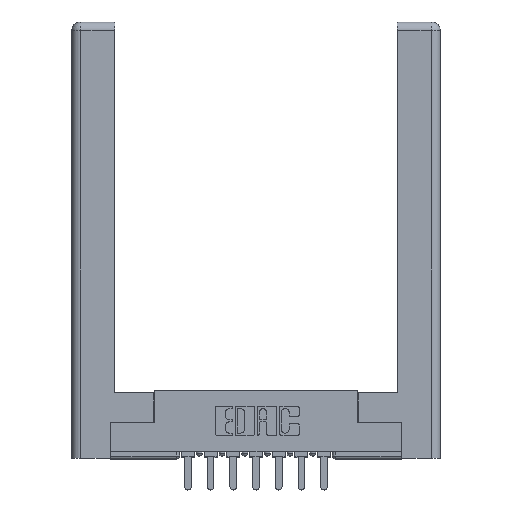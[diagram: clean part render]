
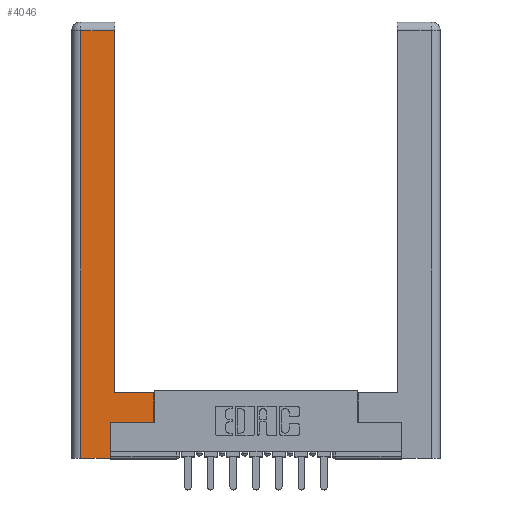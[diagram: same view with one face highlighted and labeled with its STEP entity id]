
A CAD part, top view. The second image highlights one B-rep face of the part: STEP entity #4046.
In plain terms, the highlighted planar face has unit normal (0, 0, 1).
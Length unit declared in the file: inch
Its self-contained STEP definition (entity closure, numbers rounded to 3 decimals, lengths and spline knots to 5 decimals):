
#671 = CARTESIAN_POINT ( 'NONE',  ( 0., 0., 0. ) ) ;
#1032 = VECTOR ( 'NONE', #11446, 39.37008 ) ;
#1261 = VERTEX_POINT ( 'NONE', #8111 ) ;
#1289 = EDGE_CURVE ( 'NONE', #1261, #2173, #3380, .T. ) ;
#1512 = CARTESIAN_POINT ( 'NONE',  ( 0.565, 0.45, 0. ) ) ;
#1563 = FACE_OUTER_BOUND ( 'NONE', #9582, .T. ) ;
#2034 = CARTESIAN_POINT ( 'NONE',  ( 0.565, 0.245, 0. ) ) ;
#2173 = VERTEX_POINT ( 'NONE', #6510 ) ;
#2252 = VERTEX_POINT ( 'NONE', #1512 ) ;
#2338 = ORIENTED_EDGE ( 'NONE', *, *, #1289, .T. ) ;
#2406 = ORIENTED_EDGE ( 'NONE', *, *, #3808, .T. ) ;
#2448 = ORIENTED_EDGE ( 'NONE', *, *, #5752, .T. ) ;
#2510 = LINE ( 'NONE', #8804, #9296 ) ;
#2558 = DIRECTION ( 'NONE',  ( -1., 0., 0. ) ) ;
#2727 = LINE ( 'NONE', #11170, #12758 ) ;
#3006 = LINE ( 'NONE', #4801, #8708 ) ;
#3030 = ORIENTED_EDGE ( 'NONE', *, *, #5508, .T. ) ;
#3164 = VECTOR ( 'NONE', #12103, 39.37008 ) ;
#3380 = LINE ( 'NONE', #12599, #9649 ) ;
#3808 = EDGE_CURVE ( 'NONE', #2252, #13091, #12413, .T. ) ;
#4046 = ADVANCED_FACE ( 'NONE', ( #1563 ), #8781, .F. ) ;
#4602 = CARTESIAN_POINT ( 'NONE',  ( 0.295, 0.45, 0. ) ) ;
#4801 = CARTESIAN_POINT ( 'NONE',  ( 0.0615, 2.94, 0. ) ) ;
#5063 = DIRECTION ( 'NONE',  ( 0., -1., 0. ) ) ;
#5065 = DIRECTION ( 'NONE',  ( 1., 0., 0. ) ) ;
#5245 = EDGE_CURVE ( 'NONE', #2173, #11955, #7089, .T. ) ;
#5508 = EDGE_CURVE ( 'NONE', #11955, #2252, #2510, .T. ) ;
#5752 = EDGE_CURVE ( 'NONE', #6782, #6226, #2727, .T. ) ;
#6035 = CARTESIAN_POINT ( 'NONE',  ( 0.265, 0., 0. ) ) ;
#6226 = VERTEX_POINT ( 'NONE', #11432 ) ;
#6386 = CARTESIAN_POINT ( 'NONE',  ( 0.0615, 2.94, 0. ) ) ;
#6510 = CARTESIAN_POINT ( 'NONE',  ( 0.265, 0.245, 0. ) ) ;
#6622 = CARTESIAN_POINT ( 'NONE',  ( 0.295, 3., 0. ) ) ;
#6713 = ORIENTED_EDGE ( 'NONE', *, *, #10394, .T. ) ;
#6782 = VERTEX_POINT ( 'NONE', #6386 ) ;
#6905 = DIRECTION ( 'NONE',  ( 0., 0., -1. ) ) ;
#7023 = EDGE_CURVE ( 'NONE', #6226, #1261, #11310, .T. ) ;
#7089 = LINE ( 'NONE', #2034, #7773 ) ;
#7704 = AXIS2_PLACEMENT_3D ( 'NONE', #671, #6905, #2558 ) ;
#7773 = VECTOR ( 'NONE', #11322, 39.37008 ) ;
#7911 = CARTESIAN_POINT ( 'NONE',  ( 0.565, 0.245, 0. ) ) ;
#7975 = CARTESIAN_POINT ( 'NONE',  ( 0.295, 2.94, 0. ) ) ;
#7979 = DIRECTION ( 'NONE',  ( 0., 1., 0. ) ) ;
#8111 = CARTESIAN_POINT ( 'NONE',  ( 0.265, 0., 0. ) ) ;
#8347 = ORIENTED_EDGE ( 'NONE', *, *, #5245, .T. ) ;
#8708 = VECTOR ( 'NONE', #13468, 39.37008 ) ;
#8781 = PLANE ( 'NONE',  #7704 ) ;
#8804 = CARTESIAN_POINT ( 'NONE',  ( 0.565, 0.45, 0. ) ) ;
#9127 = EDGE_CURVE ( 'NONE', #13091, #10915, #11062, .T. ) ;
#9296 = VECTOR ( 'NONE', #7979, 39.37008 ) ;
#9582 = EDGE_LOOP ( 'NONE', ( #9651, #6713, #2448, #11566, #2338, #8347, #3030, #2406 ) ) ;
#9649 = VECTOR ( 'NONE', #12734, 39.37008 ) ;
#9651 = ORIENTED_EDGE ( 'NONE', *, *, #9127, .T. ) ;
#10394 = EDGE_CURVE ( 'NONE', #10915, #6782, #3006, .T. ) ;
#10407 = VECTOR ( 'NONE', #5065, 39.37008 ) ;
#10915 = VERTEX_POINT ( 'NONE', #7975 ) ;
#11062 = LINE ( 'NONE', #6622, #3164 ) ;
#11170 = CARTESIAN_POINT ( 'NONE',  ( 0.0615, 0., 0. ) ) ;
#11310 = LINE ( 'NONE', #6035, #10407 ) ;
#11322 = DIRECTION ( 'NONE',  ( 1., 0., 0. ) ) ;
#11432 = CARTESIAN_POINT ( 'NONE',  ( 0.0615, 0., 0. ) ) ;
#11446 = DIRECTION ( 'NONE',  ( -1., 0., 0. ) ) ;
#11566 = ORIENTED_EDGE ( 'NONE', *, *, #7023, .T. ) ;
#11955 = VERTEX_POINT ( 'NONE', #7911 ) ;
#12103 = DIRECTION ( 'NONE',  ( 0., 1., 0. ) ) ;
#12413 = LINE ( 'NONE', #12477, #1032 ) ;
#12477 = CARTESIAN_POINT ( 'NONE',  ( 0.295, 0.45, 0. ) ) ;
#12599 = CARTESIAN_POINT ( 'NONE',  ( 0.265, 0.245, 0. ) ) ;
#12734 = DIRECTION ( 'NONE',  ( 0., 1., 0. ) ) ;
#12758 = VECTOR ( 'NONE', #5063, 39.37008 ) ;
#13091 = VERTEX_POINT ( 'NONE', #4602 ) ;
#13468 = DIRECTION ( 'NONE',  ( -1., 0., 0. ) ) ;
